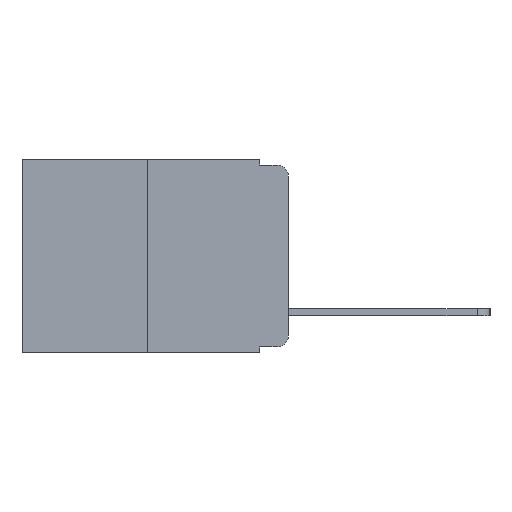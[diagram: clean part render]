
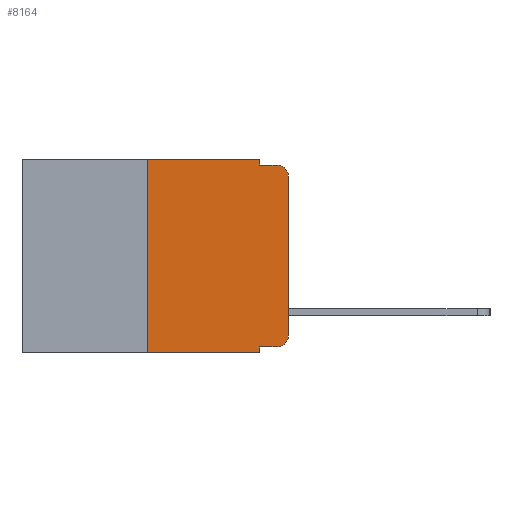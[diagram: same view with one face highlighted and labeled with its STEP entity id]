
A CAD part, left-side view. The second image highlights one B-rep face of the part: STEP entity #8164.
In plain terms, the highlighted planar face has unit normal (-1, 0, 0).
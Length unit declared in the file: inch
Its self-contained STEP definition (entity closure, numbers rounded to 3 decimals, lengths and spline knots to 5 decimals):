
#40 = CARTESIAN_POINT ( 'NONE',  ( 0., 0.051, 0. ) ) ;
#484 = CARTESIAN_POINT ( 'NONE',  ( 0., 0.051, -0.333 ) ) ;
#909 = ORIENTED_EDGE ( 'NONE', *, *, #3162, .F. ) ;
#1035 = VECTOR ( 'NONE', #6275, 39.37008 ) ;
#1272 = ORIENTED_EDGE ( 'NONE', *, *, #4142, .F. ) ;
#1293 = VECTOR ( 'NONE', #10456, 39.37008 ) ;
#1364 = VERTEX_POINT ( 'NONE', #12476 ) ;
#1609 = CARTESIAN_POINT ( 'NONE',  ( 0., 0.473, 0. ) ) ;
#1648 = EDGE_LOOP ( 'NONE', ( #3176, #6123, #909, #3889, #1272, #12609, #4556, #7491, #1996, #4871 ) ) ;
#1660 = LINE ( 'NONE', #13223, #3544 ) ;
#1699 = EDGE_CURVE ( 'NONE', #4708, #3780, #13252, .T. ) ;
#1896 = AXIS2_PLACEMENT_3D ( 'NONE', #9652, #9615, #9612 ) ;
#1996 = ORIENTED_EDGE ( 'NONE', *, *, #6134, .T. ) ;
#2140 = CARTESIAN_POINT ( 'NONE',  ( 0., 0.051, 0. ) ) ;
#2311 = CARTESIAN_POINT ( 'NONE',  ( 0., 0.051, -0.01 ) ) ;
#2409 = EDGE_CURVE ( 'NONE', #3780, #1364, #10912, .T. ) ;
#2497 = CARTESIAN_POINT ( 'NONE',  ( 0., 0., -0.03 ) ) ;
#2879 = DIRECTION ( 'NONE',  ( 0., -1., 0. ) ) ;
#2906 = VERTEX_POINT ( 'NONE', #8707 ) ;
#2978 = LINE ( 'NONE', #10885, #8486 ) ;
#3120 = CARTESIAN_POINT ( 'NONE',  ( 0., 0.02, -0.333 ) ) ;
#3162 = EDGE_CURVE ( 'NONE', #8024, #1364, #1660, .T. ) ;
#3176 = ORIENTED_EDGE ( 'NONE', *, *, #1699, .T. ) ;
#3531 = VERTEX_POINT ( 'NONE', #9439 ) ;
#3544 = VECTOR ( 'NONE', #9190, 39.37008 ) ;
#3780 = VERTEX_POINT ( 'NONE', #2497 ) ;
#3889 = ORIENTED_EDGE ( 'NONE', *, *, #3921, .F. ) ;
#3921 = EDGE_CURVE ( 'NONE', #4704, #8024, #7159, .T. ) ;
#3925 = VERTEX_POINT ( 'NONE', #8031 ) ;
#4060 = VECTOR ( 'NONE', #5178, 39.37008 ) ;
#4142 = EDGE_CURVE ( 'NONE', #8886, #4704, #12764, .T. ) ;
#4341 = CIRCLE ( 'NONE', #1896, 0.02 ) ;
#4392 = LINE ( 'NONE', #8679, #4060 ) ;
#4556 = ORIENTED_EDGE ( 'NONE', *, *, #4982, .T. ) ;
#4624 = CARTESIAN_POINT ( 'NONE',  ( 0., 0., 0. ) ) ;
#4631 = EDGE_CURVE ( 'NONE', #3531, #8886, #4392, .T. ) ;
#4704 = VERTEX_POINT ( 'NONE', #2140 ) ;
#4708 = VERTEX_POINT ( 'NONE', #9080 ) ;
#4871 = ORIENTED_EDGE ( 'NONE', *, *, #6869, .T. ) ;
#4982 = EDGE_CURVE ( 'NONE', #3531, #3925, #2978, .T. ) ;
#5178 = DIRECTION ( 'NONE',  ( 0., 0., 1. ) ) ;
#5373 = EDGE_CURVE ( 'NONE', #2906, #3925, #6935, .T. ) ;
#5893 = CARTESIAN_POINT ( 'NONE',  ( 0., 0.473, 0. ) ) ;
#5970 = VERTEX_POINT ( 'NONE', #3120 ) ;
#6123 = ORIENTED_EDGE ( 'NONE', *, *, #2409, .T. ) ;
#6134 = EDGE_CURVE ( 'NONE', #2906, #5970, #12077, .T. ) ;
#6275 = DIRECTION ( 'NONE',  ( 0., 0., -1. ) ) ;
#6391 = DIRECTION ( 'NONE',  ( 0., 0., -1. ) ) ;
#6467 = DIRECTION ( 'NONE',  ( 0., 0., 1. ) ) ;
#6572 = VECTOR ( 'NONE', #7303, 39.37008 ) ;
#6869 = EDGE_CURVE ( 'NONE', #5970, #4708, #4341, .T. ) ;
#6935 = LINE ( 'NONE', #11072, #1035 ) ;
#6987 = DIRECTION ( 'NONE',  ( 0., 0., -1. ) ) ;
#7148 = AXIS2_PLACEMENT_3D ( 'NONE', #5893, #13115, #6987 ) ;
#7159 = LINE ( 'NONE', #40, #1293 ) ;
#7303 = DIRECTION ( 'NONE',  ( 0., -1., 0. ) ) ;
#7491 = ORIENTED_EDGE ( 'NONE', *, *, #5373, .F. ) ;
#8024 = VERTEX_POINT ( 'NONE', #2311 ) ;
#8031 = CARTESIAN_POINT ( 'NONE',  ( 0., 0.051, -0.343 ) ) ;
#8164 = ADVANCED_FACE ( 'NONE', ( #10947 ), #10108, .F. ) ;
#8402 = CARTESIAN_POINT ( 'NONE',  ( 0., 0.02, -0.03 ) ) ;
#8486 = VECTOR ( 'NONE', #2879, 39.37008 ) ;
#8679 = CARTESIAN_POINT ( 'NONE',  ( 0., 0.25, 0. ) ) ;
#8707 = CARTESIAN_POINT ( 'NONE',  ( 0., 0.051, -0.333 ) ) ;
#8886 = VERTEX_POINT ( 'NONE', #10345 ) ;
#9080 = CARTESIAN_POINT ( 'NONE',  ( 0., 0., -0.313 ) ) ;
#9190 = DIRECTION ( 'NONE',  ( 0., -1., 0. ) ) ;
#9439 = CARTESIAN_POINT ( 'NONE',  ( 0., 0.25, -0.343 ) ) ;
#9481 = AXIS2_PLACEMENT_3D ( 'NONE', #8402, #12756, #6391 ) ;
#9612 = DIRECTION ( 'NONE',  ( 0., 0., -1. ) ) ;
#9615 = DIRECTION ( 'NONE',  ( -1., 0., 0. ) ) ;
#9652 = CARTESIAN_POINT ( 'NONE',  ( 0., 0.02, -0.313 ) ) ;
#9784 = VECTOR ( 'NONE', #9845, 39.37008 ) ;
#9845 = DIRECTION ( 'NONE',  ( 0., -1., 0. ) ) ;
#10108 = PLANE ( 'NONE',  #7148 ) ;
#10345 = CARTESIAN_POINT ( 'NONE',  ( 0., 0.25, 0. ) ) ;
#10456 = DIRECTION ( 'NONE',  ( 0., 0., -1. ) ) ;
#10598 = VECTOR ( 'NONE', #6467, 39.37008 ) ;
#10885 = CARTESIAN_POINT ( 'NONE',  ( 0., 0.473, -0.343 ) ) ;
#10912 = CIRCLE ( 'NONE', #9481, 0.02 ) ;
#10947 = FACE_OUTER_BOUND ( 'NONE', #1648, .T. ) ;
#11072 = CARTESIAN_POINT ( 'NONE',  ( 0., 0.051, 0. ) ) ;
#12077 = LINE ( 'NONE', #484, #6572 ) ;
#12476 = CARTESIAN_POINT ( 'NONE',  ( 0., 0.02, -0.01 ) ) ;
#12609 = ORIENTED_EDGE ( 'NONE', *, *, #4631, .F. ) ;
#12756 = DIRECTION ( 'NONE',  ( -1., 0., 0. ) ) ;
#12764 = LINE ( 'NONE', #1609, #9784 ) ;
#13115 = DIRECTION ( 'NONE',  ( 1., 0., 0. ) ) ;
#13223 = CARTESIAN_POINT ( 'NONE',  ( 0., 0.051, -0.01 ) ) ;
#13252 = LINE ( 'NONE', #4624, #10598 ) ;
